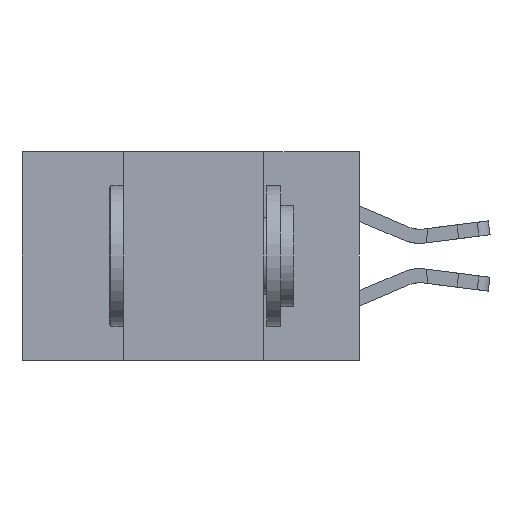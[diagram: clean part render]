
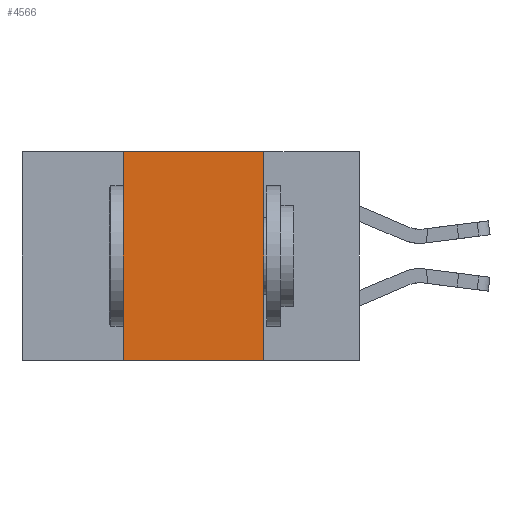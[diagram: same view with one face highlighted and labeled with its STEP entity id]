
A CAD part, left-side view. The second image highlights one B-rep face of the part: STEP entity #4566.
In plain terms, the highlighted planar face has unit normal (-1, 0, 0).
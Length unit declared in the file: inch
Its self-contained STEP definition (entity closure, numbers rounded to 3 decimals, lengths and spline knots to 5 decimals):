
#501 = DIRECTION ( 'NONE',  ( 0., 0., -1. ) ) ;
#2261 = DIRECTION ( 'NONE',  ( 0., -1., 0. ) ) ;
#3327 = VERTEX_POINT ( 'NONE', #18999 ) ;
#4566 = ADVANCED_FACE ( 'NONE', ( #26983 ), #25468, .F. ) ;
#5563 = DIRECTION ( 'NONE',  ( 1., 0., 0. ) ) ;
#6543 = ORIENTED_EDGE ( 'NONE', *, *, #26437, .T. ) ;
#6881 = VECTOR ( 'NONE', #10148, 39.37008 ) ;
#6913 = CARTESIAN_POINT ( 'NONE',  ( 0., 0.6, 0. ) ) ;
#7080 = CARTESIAN_POINT ( 'NONE',  ( 0., 0.17, 0. ) ) ;
#7776 = ORIENTED_EDGE ( 'NONE', *, *, #22481, .F. ) ;
#7922 = DIRECTION ( 'NONE',  ( 0., 0., -1. ) ) ;
#10148 = DIRECTION ( 'NONE',  ( 0., 0., 1. ) ) ;
#11763 = VECTOR ( 'NONE', #501, 39.37008 ) ;
#12037 = LINE ( 'NONE', #6913, #14858 ) ;
#12894 = LINE ( 'NONE', #19017, #6881 ) ;
#14639 = CARTESIAN_POINT ( 'NONE',  ( 0., 0.17, 0. ) ) ;
#14858 = VECTOR ( 'NONE', #2261, 39.37008 ) ;
#15163 = AXIS2_PLACEMENT_3D ( 'NONE', #16897, #5563, #7922 ) ;
#16001 = EDGE_CURVE ( 'NONE', #24542, #27474, #22548, .T. ) ;
#16897 = CARTESIAN_POINT ( 'NONE',  ( 0., 0.6, 0. ) ) ;
#16984 = ORIENTED_EDGE ( 'NONE', *, *, #20165, .F. ) ;
#17823 = DIRECTION ( 'NONE',  ( 0., -1., 0. ) ) ;
#18178 = VERTEX_POINT ( 'NONE', #28146 ) ;
#18999 = CARTESIAN_POINT ( 'NONE',  ( 0., 0.42, 0. ) ) ;
#19017 = CARTESIAN_POINT ( 'NONE',  ( 0., 0.42, 0. ) ) ;
#19881 = CARTESIAN_POINT ( 'NONE',  ( 0., 0.6, -0.37 ) ) ;
#20165 = EDGE_CURVE ( 'NONE', #18178, #3327, #12894, .T. ) ;
#20302 = LINE ( 'NONE', #19881, #25542 ) ;
#21415 = CARTESIAN_POINT ( 'NONE',  ( 0., 0.17, -0.37 ) ) ;
#22481 = EDGE_CURVE ( 'NONE', #3327, #24542, #12037, .T. ) ;
#22548 = LINE ( 'NONE', #7080, #11763 ) ;
#24542 = VERTEX_POINT ( 'NONE', #14639 ) ;
#25468 = PLANE ( 'NONE',  #15163 ) ;
#25542 = VECTOR ( 'NONE', #17823, 39.37008 ) ;
#26432 = EDGE_LOOP ( 'NONE', ( #27134, #7776, #16984, #6543 ) ) ;
#26437 = EDGE_CURVE ( 'NONE', #18178, #27474, #20302, .T. ) ;
#26983 = FACE_OUTER_BOUND ( 'NONE', #26432, .T. ) ;
#27134 = ORIENTED_EDGE ( 'NONE', *, *, #16001, .F. ) ;
#27474 = VERTEX_POINT ( 'NONE', #21415 ) ;
#28146 = CARTESIAN_POINT ( 'NONE',  ( 0., 0.42, -0.37 ) ) ;
